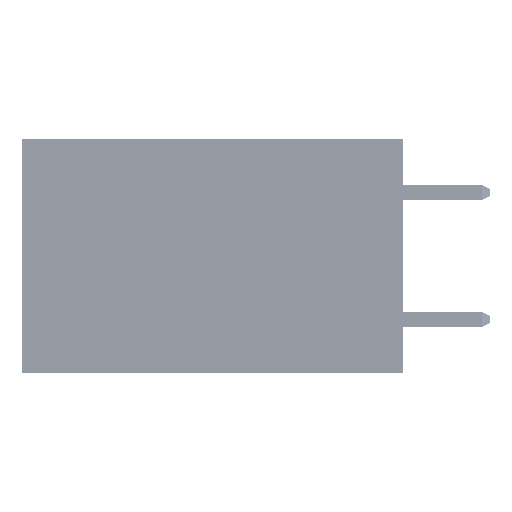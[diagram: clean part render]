
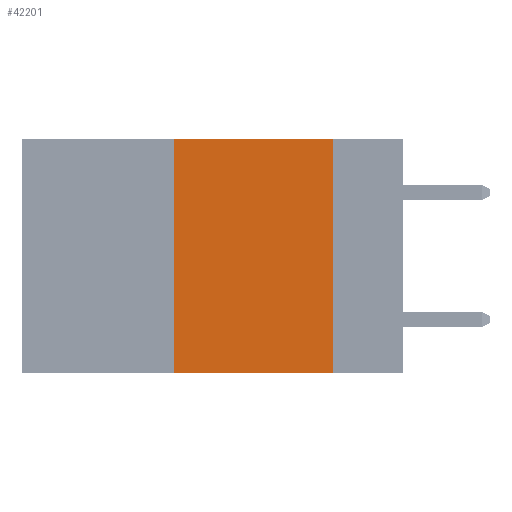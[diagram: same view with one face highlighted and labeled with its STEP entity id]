
A CAD part, left-side view. The second image highlights one B-rep face of the part: STEP entity #42201.
In plain terms, the highlighted planar face has unit normal (-1, 0, 0).
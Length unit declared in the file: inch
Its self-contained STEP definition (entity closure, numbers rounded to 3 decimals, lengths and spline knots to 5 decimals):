
#553 = DIRECTION ( 'NONE',  ( 0., 0., -1. ) ) ;
#4342 = LINE ( 'NONE', #19674, #34579 ) ;
#6998 = ORIENTED_EDGE ( 'NONE', *, *, #18728, .F. ) ;
#7537 = DIRECTION ( 'NONE',  ( 0., 0., 1. ) ) ;
#8868 = LINE ( 'NONE', #31829, #48090 ) ;
#12390 = VECTOR ( 'NONE', #47666, 39.37008 ) ;
#12654 = DIRECTION ( 'NONE',  ( 0., -1., 0. ) ) ;
#13101 = EDGE_CURVE ( 'NONE', #45703, #36498, #4342, .T. ) ;
#15313 = FACE_OUTER_BOUND ( 'NONE', #44074, .T. ) ;
#16032 = AXIS2_PLACEMENT_3D ( 'NONE', #21908, #37312, #18852 ) ;
#18728 = EDGE_CURVE ( 'NONE', #20864, #45703, #24935, .T. ) ;
#18852 = DIRECTION ( 'NONE',  ( 0., 0., -1. ) ) ;
#19674 = CARTESIAN_POINT ( 'NONE',  ( 0., 0.11, 0. ) ) ;
#19684 = CARTESIAN_POINT ( 'NONE',  ( 0., 0.36, -0.37 ) ) ;
#20864 = VERTEX_POINT ( 'NONE', #21517 ) ;
#21517 = CARTESIAN_POINT ( 'NONE',  ( 0., 0.36, 0. ) ) ;
#21908 = CARTESIAN_POINT ( 'NONE',  ( 0., 0.6, 0. ) ) ;
#23531 = EDGE_CURVE ( 'NONE', #31467, #36498, #8868, .T. ) ;
#24935 = LINE ( 'NONE', #43627, #12390 ) ;
#25653 = EDGE_CURVE ( 'NONE', #31467, #20864, #27687, .T. ) ;
#27687 = LINE ( 'NONE', #45885, #40379 ) ;
#28956 = CARTESIAN_POINT ( 'NONE',  ( 0., 0.11, 0. ) ) ;
#31467 = VERTEX_POINT ( 'NONE', #19684 ) ;
#31829 = CARTESIAN_POINT ( 'NONE',  ( 0., 0.6, -0.37 ) ) ;
#33030 = ORIENTED_EDGE ( 'NONE', *, *, #23531, .T. ) ;
#33376 = CARTESIAN_POINT ( 'NONE',  ( 0., 0.11, -0.37 ) ) ;
#34579 = VECTOR ( 'NONE', #553, 39.37008 ) ;
#36498 = VERTEX_POINT ( 'NONE', #33376 ) ;
#37312 = DIRECTION ( 'NONE',  ( 1., 0., 0. ) ) ;
#38382 = ORIENTED_EDGE ( 'NONE', *, *, #25653, .F. ) ;
#40379 = VECTOR ( 'NONE', #7537, 39.37008 ) ;
#42201 = ADVANCED_FACE ( 'NONE', ( #15313 ), #45380, .F. ) ;
#43627 = CARTESIAN_POINT ( 'NONE',  ( 0., 0.6, 0. ) ) ;
#44074 = EDGE_LOOP ( 'NONE', ( #48147, #6998, #38382, #33030 ) ) ;
#45380 = PLANE ( 'NONE',  #16032 ) ;
#45703 = VERTEX_POINT ( 'NONE', #28956 ) ;
#45885 = CARTESIAN_POINT ( 'NONE',  ( 0., 0.36, 0. ) ) ;
#47666 = DIRECTION ( 'NONE',  ( 0., -1., 0. ) ) ;
#48090 = VECTOR ( 'NONE', #12654, 39.37008 ) ;
#48147 = ORIENTED_EDGE ( 'NONE', *, *, #13101, .F. ) ;
